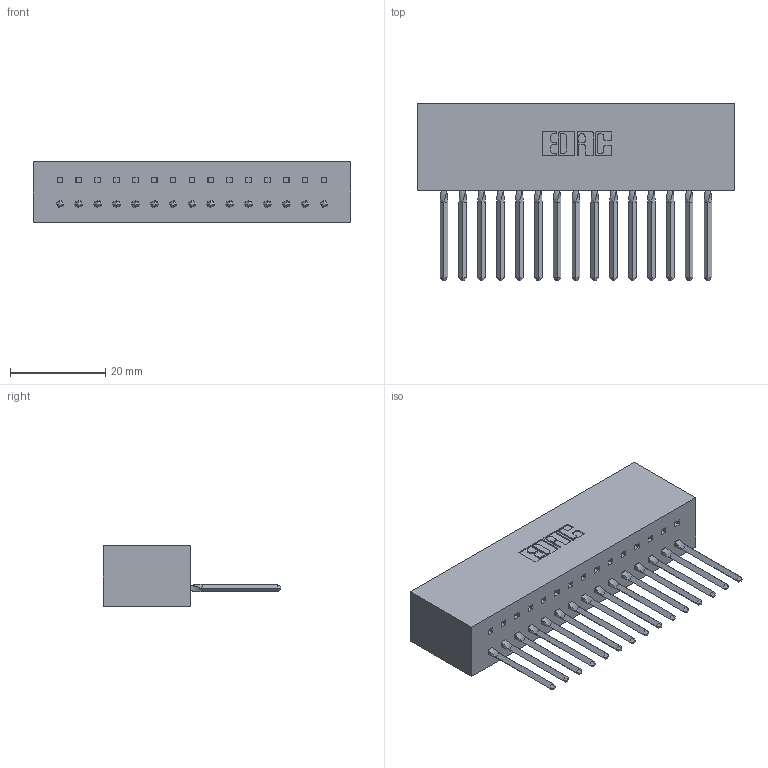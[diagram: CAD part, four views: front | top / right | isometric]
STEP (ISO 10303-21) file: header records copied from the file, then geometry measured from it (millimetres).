
FILE_DESCRIPTION (( 'STEP AP203' ), '1' );
FILE_NAME ('317-015-541-601.STEP', '2020-02-27T15:02:03', ( '' ), ( '' ), 'SwSTEP 2.0', 'SolidWorks 2016', '' );
FILE_SCHEMA (( 'CONFIG_CONTROL_DESIGN' ));
Length unit declared in the file: inch
Products named in the file (3): 317-015-541-601; 317 Part_Lugless; 317-290-002_541
Assembly tree (16 placements, depth 2):
  317-015-541-601
    317 Part_Lugless
    317-290-002_541  x15
Bounding box: 66.65 x 37.34 x 12.7 mm (x, y, z)
Volume: 11683.9 mm3; surface area: 15803.7 mm2
Topology: 16 solids, 16 shells, 2370 faces, 6749 edges, 4388 vertices
Faces by surface type: plane 1910, cylinder 400, bspline 60
Entity records: 26108 total; most frequent: CARTESIAN_POINT 5270, ORIENTED_EDGE 4538, DIRECTION 3699, EDGE_CURVE 2269, VECTOR 1913, LINE 1913, VERTEX_POINT 1504, AXIS2_PLACEMENT_3D 893
